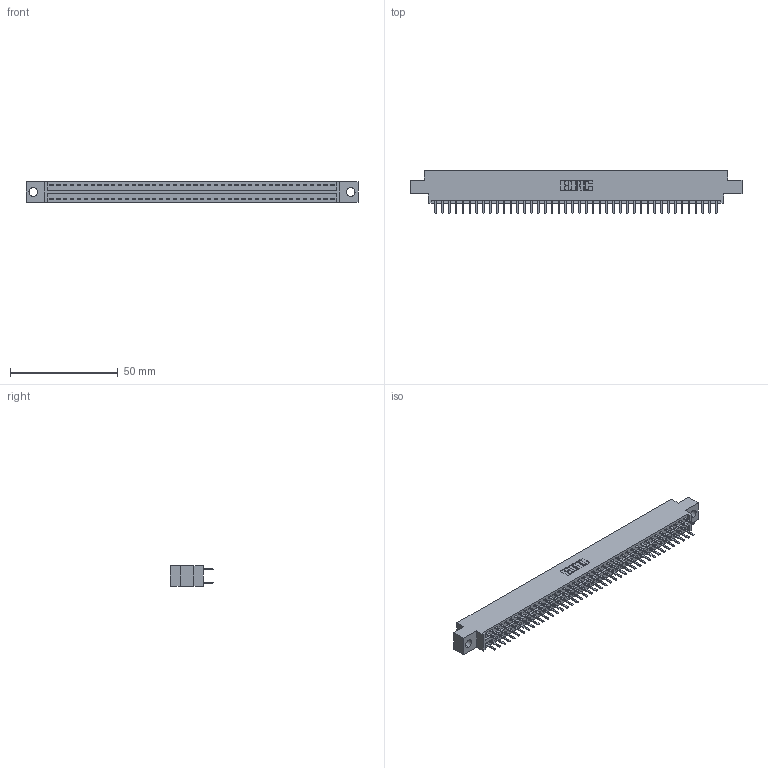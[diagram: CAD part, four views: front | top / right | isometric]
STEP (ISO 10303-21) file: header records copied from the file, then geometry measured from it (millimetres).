
FILE_DESCRIPTION (( 'STEP AP203' ), '1' );
FILE_NAME ('346-084-520-804.STEP', '2022-05-25T19:22:09', ( '' ), ( '' ), 'SwSTEP 2.0', 'SolidWorks 2020', '' );
FILE_SCHEMA (( 'CONFIG_CONTROL_DESIGN' ));
Length unit declared in the file: inch
Products named in the file (3): 346-084-520-804; 345-292-001_345-293-120; 346 Part_0.170 Offset - 0.156 Dia-TH
Assembly tree (85 placements, depth 2):
  346-084-520-804
    346 Part_0.170 Offset - 0.156 Dia-TH
    345-292-001_345-293-120  x84
Bounding box: 153.92 x 20.02 x 9.4 mm (x, y, z)
Volume: 14712 mm3; surface area: 20163.6 mm2
Topology: 85 solids, 85 shells, 4844 faces, 14069 edges, 9154 vertices
Faces by surface type: plane 3202, cylinder 1642
Entity records: 28075 total; most frequent: CARTESIAN_POINT 4646, ORIENTED_EDGE 4566, DIRECTION 4131, EDGE_CURVE 2283, LINE 1979, VECTOR 1979, VERTEX_POINT 1518, AXIS2_PLACEMENT_3D 1076
